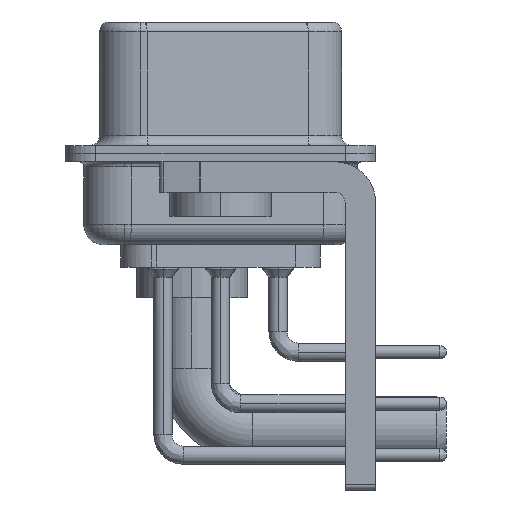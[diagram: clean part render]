
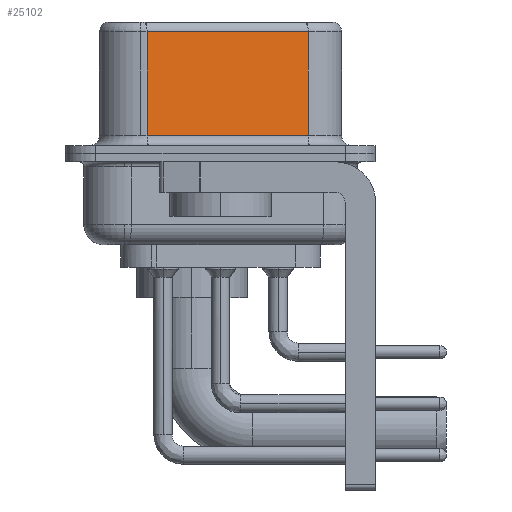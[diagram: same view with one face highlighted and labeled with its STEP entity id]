
A CAD part, left-side view. The second image highlights one B-rep face of the part: STEP entity #25102.
In plain terms, the highlighted planar face has unit normal (-0.985, -0.174, 0).
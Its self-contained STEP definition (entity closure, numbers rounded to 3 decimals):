
#247 = LINE ( 'NONE', #26452, #5086 ) ;
#673 = LINE ( 'NONE', #15413, #11702 ) ;
#1761 = VERTEX_POINT ( 'NONE', #30537 ) ;
#4122 = EDGE_LOOP ( 'NONE', ( #21479, #16905, #34977, #24428 ) ) ;
#5066 = CARTESIAN_POINT ( 'NONE',  ( 3.73, 3.628, 0.9 ) ) ;
#5086 = VECTOR ( 'NONE', #17885, 1000. ) ;
#5608 = VECTOR ( 'NONE', #26666, 1000. ) ;
#8822 = CARTESIAN_POINT ( 'NONE',  ( 3.73, 3.628, 6.52 ) ) ;
#9195 = LINE ( 'NONE', #8822, #5608 ) ;
#9512 = EDGE_CURVE ( 'NONE', #28556, #20218, #9195, .T. ) ;
#11271 = EDGE_CURVE ( 'NONE', #20218, #13641, #247, .T. ) ;
#11702 = VECTOR ( 'NONE', #36383, 1000. ) ;
#13641 = VERTEX_POINT ( 'NONE', #22255 ) ;
#15413 = CARTESIAN_POINT ( 'NONE',  ( 5.132, -4.322, 6.52 ) ) ;
#16205 = FACE_OUTER_BOUND ( 'NONE', #4122, .T. ) ;
#16905 = ORIENTED_EDGE ( 'NONE', *, *, #25987, .T. ) ;
#17008 = AXIS2_PLACEMENT_3D ( 'NONE', #19876, #19119, #28839 ) ;
#17885 = DIRECTION ( 'NONE',  ( 0.174, -0.985, 0. ) ) ;
#18455 = DIRECTION ( 'NONE',  ( -0.174, 0.985, 0. ) ) ;
#19119 = DIRECTION ( 'NONE',  ( 0.985, 0.174, 0. ) ) ;
#19362 = EDGE_CURVE ( 'NONE', #1761, #13641, #673, .T. ) ;
#19876 = CARTESIAN_POINT ( 'NONE',  ( 5.132, -4.322, 6.52 ) ) ;
#20218 = VERTEX_POINT ( 'NONE', #5066 ) ;
#21479 = ORIENTED_EDGE ( 'NONE', *, *, #19362, .F. ) ;
#22255 = CARTESIAN_POINT ( 'NONE',  ( 5.132, -4.322, 0.9 ) ) ;
#22621 = PLANE ( 'NONE',  #17008 ) ;
#22641 = VECTOR ( 'NONE', #18455, 1000. ) ;
#24428 = ORIENTED_EDGE ( 'NONE', *, *, #11271, .T. ) ;
#25102 = ADVANCED_FACE ( 'NONE', ( #16205 ), #22621, .F. ) ;
#25360 = CARTESIAN_POINT ( 'NONE',  ( 3.73, 3.628, 6.02 ) ) ;
#25987 = EDGE_CURVE ( 'NONE', #1761, #28556, #36139, .T. ) ;
#26452 = CARTESIAN_POINT ( 'NONE',  ( 5.132, -4.322, 0.9 ) ) ;
#26666 = DIRECTION ( 'NONE',  ( 0., 0., -1. ) ) ;
#28556 = VERTEX_POINT ( 'NONE', #25360 ) ;
#28839 = DIRECTION ( 'NONE',  ( -0.174, 0.985, 0. ) ) ;
#30537 = CARTESIAN_POINT ( 'NONE',  ( 5.132, -4.322, 6.02 ) ) ;
#33240 = CARTESIAN_POINT ( 'NONE',  ( 5.132, -4.322, 6.02 ) ) ;
#34977 = ORIENTED_EDGE ( 'NONE', *, *, #9512, .T. ) ;
#36139 = LINE ( 'NONE', #33240, #22641 ) ;
#36383 = DIRECTION ( 'NONE',  ( 0., 0., -1. ) ) ;
